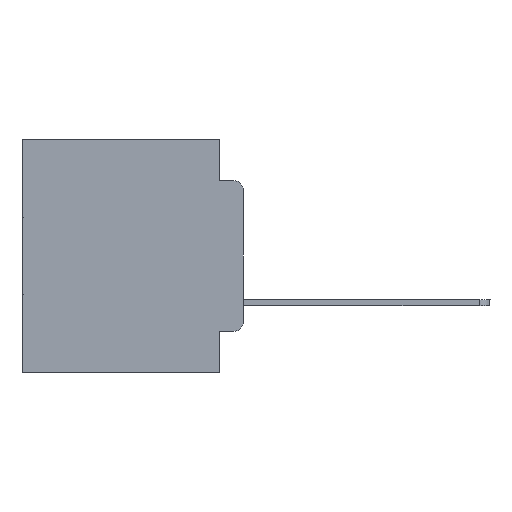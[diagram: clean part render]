
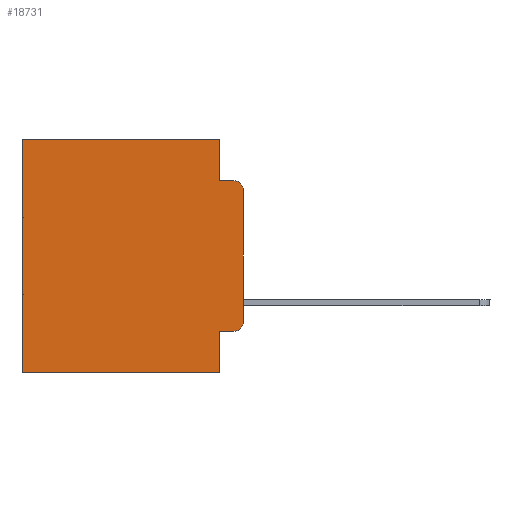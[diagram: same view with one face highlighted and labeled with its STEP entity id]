
A CAD part, left-side view. The second image highlights one B-rep face of the part: STEP entity #18731.
In plain terms, the highlighted planar face has unit normal (-1, 0, 0).
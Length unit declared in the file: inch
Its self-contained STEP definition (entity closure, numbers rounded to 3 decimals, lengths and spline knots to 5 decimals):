
#120 = VECTOR ( 'NONE', #6530, 39.37008 ) ;
#489 = LINE ( 'NONE', #2773, #751 ) ;
#751 = VECTOR ( 'NONE', #11958, 39.37008 ) ;
#1203 = DIRECTION ( 'NONE',  ( 0., 0., -1. ) ) ;
#2314 = ORIENTED_EDGE ( 'NONE', *, *, #9898, .T. ) ;
#2773 = CARTESIAN_POINT ( 'NONE',  ( 0.298, 0., 0. ) ) ;
#2982 = AXIS2_PLACEMENT_3D ( 'NONE', #24264, #12215, #1203 ) ;
#3006 = LINE ( 'NONE', #18987, #11737 ) ;
#3108 = EDGE_CURVE ( 'NONE', #4319, #15697, #489, .T. ) ;
#3141 = CARTESIAN_POINT ( 'NONE',  ( 0.298, 0., 0. ) ) ;
#3705 = VERTEX_POINT ( 'NONE', #20209 ) ;
#3821 = DIRECTION ( 'NONE',  ( 0., 0., -1. ) ) ;
#4021 = LINE ( 'NONE', #18045, #15818 ) ;
#4319 = VERTEX_POINT ( 'NONE', #18201 ) ;
#6522 = CARTESIAN_POINT ( 'NONE',  ( 0.298, 0.473, 0. ) ) ;
#6530 = DIRECTION ( 'NONE',  ( 0., 0., -1. ) ) ;
#6637 = VERTEX_POINT ( 'NONE', #27506 ) ;
#6826 = CARTESIAN_POINT ( 'NONE',  ( 0.298, 0.051, -0.0885 ) ) ;
#6898 = VECTOR ( 'NONE', #13903, 39.37008 ) ;
#7270 = EDGE_CURVE ( 'NONE', #9102, #9525, #28672, .T. ) ;
#7306 = CIRCLE ( 'NONE', #2982, 0.02 ) ;
#7427 = CARTESIAN_POINT ( 'NONE',  ( 0.298, 0., -0.5 ) ) ;
#7532 = DIRECTION ( 'NONE',  ( 0., 0., -1. ) ) ;
#8475 = LINE ( 'NONE', #19661, #25255 ) ;
#9102 = VERTEX_POINT ( 'NONE', #15452 ) ;
#9525 = VERTEX_POINT ( 'NONE', #6522 ) ;
#9591 = VECTOR ( 'NONE', #26848, 39.37008 ) ;
#9898 = EDGE_CURVE ( 'NONE', #26371, #15697, #7306, .T. ) ;
#10384 = ORIENTED_EDGE ( 'NONE', *, *, #13786, .F. ) ;
#10536 = CARTESIAN_POINT ( 'NONE',  ( 0.298, 0.02, -0.4115 ) ) ;
#11313 = CARTESIAN_POINT ( 'NONE',  ( 0.298, 0.051, -0.0885 ) ) ;
#11461 = ORIENTED_EDGE ( 'NONE', *, *, #7270, .T. ) ;
#11614 = DIRECTION ( 'NONE',  ( -1., 0., 0. ) ) ;
#11616 = DIRECTION ( 'NONE',  ( 0., -1., 0. ) ) ;
#11737 = VECTOR ( 'NONE', #7532, 39.37008 ) ;
#11874 = PLANE ( 'NONE',  #26849 ) ;
#11958 = DIRECTION ( 'NONE',  ( 0., 0., -1. ) ) ;
#12215 = DIRECTION ( 'NONE',  ( -1., 0., 0. ) ) ;
#12246 = AXIS2_PLACEMENT_3D ( 'NONE', #25958, #11614, #23243 ) ;
#12365 = ORIENTED_EDGE ( 'NONE', *, *, #19473, .F. ) ;
#12981 = CARTESIAN_POINT ( 'NONE',  ( 0.298, 0., 0. ) ) ;
#12982 = EDGE_CURVE ( 'NONE', #9525, #3705, #24902, .T. ) ;
#13153 = EDGE_CURVE ( 'NONE', #18614, #3705, #16474, .T. ) ;
#13514 = DIRECTION ( 'NONE',  ( 0., -1., 0. ) ) ;
#13786 = EDGE_CURVE ( 'NONE', #6637, #18614, #3006, .T. ) ;
#13903 = DIRECTION ( 'NONE',  ( 0., 1., 0. ) ) ;
#14604 = DIRECTION ( 'NONE',  ( 0., 0., -1. ) ) ;
#15253 = ORIENTED_EDGE ( 'NONE', *, *, #21220, .T. ) ;
#15452 = CARTESIAN_POINT ( 'NONE',  ( 0.298, 0.051, 0. ) ) ;
#15697 = VERTEX_POINT ( 'NONE', #27358 ) ;
#15818 = VECTOR ( 'NONE', #13514, 39.37008 ) ;
#15872 = CARTESIAN_POINT ( 'NONE',  ( 0.298, 0.473, 0. ) ) ;
#15999 = EDGE_CURVE ( 'NONE', #9102, #22276, #8475, .T. ) ;
#16474 = LINE ( 'NONE', #7427, #6898 ) ;
#16661 = ORIENTED_EDGE ( 'NONE', *, *, #26905, .T. ) ;
#17270 = EDGE_LOOP ( 'NONE', ( #20325, #15253, #12365, #26826, #11461, #26361, #17342, #10384, #16661, #2314 ) ) ;
#17342 = ORIENTED_EDGE ( 'NONE', *, *, #13153, .F. ) ;
#18045 = CARTESIAN_POINT ( 'NONE',  ( 0.298, 0.051, -0.4115 ) ) ;
#18085 = CARTESIAN_POINT ( 'NONE',  ( 0.298, 0.051, -0.5 ) ) ;
#18201 = CARTESIAN_POINT ( 'NONE',  ( 0.298, 0., -0.1085 ) ) ;
#18614 = VERTEX_POINT ( 'NONE', #18085 ) ;
#18731 = ADVANCED_FACE ( 'NONE', ( #25908 ), #11874, .F. ) ;
#18987 = CARTESIAN_POINT ( 'NONE',  ( 0.298, 0.051, 0. ) ) ;
#19473 = EDGE_CURVE ( 'NONE', #22276, #28185, #27459, .T. ) ;
#19661 = CARTESIAN_POINT ( 'NONE',  ( 0.298, 0.051, 0. ) ) ;
#20209 = CARTESIAN_POINT ( 'NONE',  ( 0.298, 0.473, -0.5 ) ) ;
#20325 = ORIENTED_EDGE ( 'NONE', *, *, #3108, .F. ) ;
#20424 = CIRCLE ( 'NONE', #12246, 0.02 ) ;
#21220 = EDGE_CURVE ( 'NONE', #4319, #28185, #20424, .T. ) ;
#21542 = DIRECTION ( 'NONE',  ( 1., 0., 0. ) ) ;
#22276 = VERTEX_POINT ( 'NONE', #11313 ) ;
#23243 = DIRECTION ( 'NONE',  ( 0., 0., -1. ) ) ;
#24264 = CARTESIAN_POINT ( 'NONE',  ( 0.298, 0.02, -0.3915 ) ) ;
#24902 = LINE ( 'NONE', #15872, #120 ) ;
#25255 = VECTOR ( 'NONE', #3821, 39.37008 ) ;
#25908 = FACE_OUTER_BOUND ( 'NONE', #17270, .T. ) ;
#25958 = CARTESIAN_POINT ( 'NONE',  ( 0.298, 0.02, -0.1085 ) ) ;
#26361 = ORIENTED_EDGE ( 'NONE', *, *, #12982, .T. ) ;
#26371 = VERTEX_POINT ( 'NONE', #10536 ) ;
#26826 = ORIENTED_EDGE ( 'NONE', *, *, #15999, .F. ) ;
#26848 = DIRECTION ( 'NONE',  ( 0., 1., 0. ) ) ;
#26849 = AXIS2_PLACEMENT_3D ( 'NONE', #3141, #21542, #14604 ) ;
#26905 = EDGE_CURVE ( 'NONE', #6637, #26371, #4021, .T. ) ;
#27333 = VECTOR ( 'NONE', #11616, 39.37008 ) ;
#27358 = CARTESIAN_POINT ( 'NONE',  ( 0.298, 0., -0.3915 ) ) ;
#27459 = LINE ( 'NONE', #6826, #27333 ) ;
#27506 = CARTESIAN_POINT ( 'NONE',  ( 0.298, 0.051, -0.4115 ) ) ;
#28185 = VERTEX_POINT ( 'NONE', #29217 ) ;
#28672 = LINE ( 'NONE', #12981, #9591 ) ;
#29217 = CARTESIAN_POINT ( 'NONE',  ( 0.298, 0.02, -0.0885 ) ) ;
